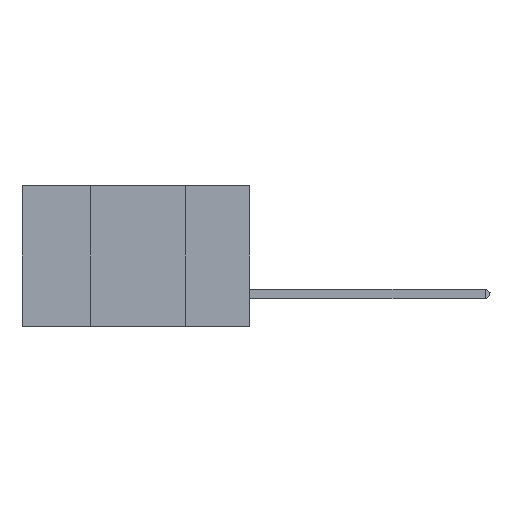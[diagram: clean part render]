
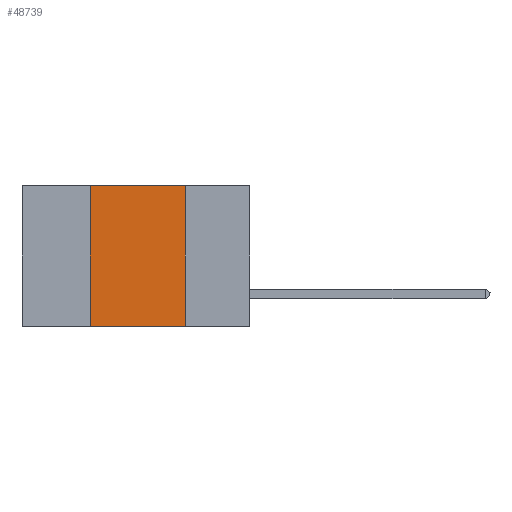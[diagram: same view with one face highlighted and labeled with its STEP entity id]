
A CAD part, left-side view. The second image highlights one B-rep face of the part: STEP entity #48739.
In plain terms, the highlighted planar face has unit normal (-1, 0, 0).
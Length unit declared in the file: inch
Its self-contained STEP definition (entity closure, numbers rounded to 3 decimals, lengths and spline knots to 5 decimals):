
#16 = LINE ( 'NONE', #6205, #40571 ) ;
#201 = CARTESIAN_POINT ( 'NONE',  ( 0., 0.6, 0. ) ) ;
#2793 = DIRECTION ( 'NONE',  ( 0., -1., 0. ) ) ;
#3436 = CARTESIAN_POINT ( 'NONE',  ( 0., 0.6, -0.37 ) ) ;
#4112 = PLANE ( 'NONE',  #21368 ) ;
#5822 = VERTEX_POINT ( 'NONE', #38594 ) ;
#6057 = ORIENTED_EDGE ( 'NONE', *, *, #24401, .F. ) ;
#6205 = CARTESIAN_POINT ( 'NONE',  ( 0., 0.6, 0. ) ) ;
#8920 = CARTESIAN_POINT ( 'NONE',  ( 0., 0.17, -0.37 ) ) ;
#11602 = CARTESIAN_POINT ( 'NONE',  ( 0., 0.17, 0. ) ) ;
#15318 = LINE ( 'NONE', #11602, #41174 ) ;
#19025 = DIRECTION ( 'NONE',  ( 0., 0., -1. ) ) ;
#19701 = VERTEX_POINT ( 'NONE', #44181 ) ;
#20139 = VERTEX_POINT ( 'NONE', #31394 ) ;
#20397 = DIRECTION ( 'NONE',  ( 1., 0., 0. ) ) ;
#21368 = AXIS2_PLACEMENT_3D ( 'NONE', #201, #20397, #40037 ) ;
#21485 = LINE ( 'NONE', #29884, #40551 ) ;
#23314 = LINE ( 'NONE', #3436, #45417 ) ;
#24401 = EDGE_CURVE ( 'NONE', #20139, #5822, #21485, .T. ) ;
#25760 = DIRECTION ( 'NONE',  ( 0., 0., 1. ) ) ;
#25845 = FACE_OUTER_BOUND ( 'NONE', #41307, .T. ) ;
#26761 = EDGE_CURVE ( 'NONE', #20139, #47123, #23314, .T. ) ;
#27064 = ORIENTED_EDGE ( 'NONE', *, *, #38876, .F. ) ;
#29884 = CARTESIAN_POINT ( 'NONE',  ( 0., 0.42, 0. ) ) ;
#31394 = CARTESIAN_POINT ( 'NONE',  ( 0., 0.42, -0.37 ) ) ;
#33507 = ORIENTED_EDGE ( 'NONE', *, *, #26761, .T. ) ;
#38249 = ORIENTED_EDGE ( 'NONE', *, *, #39695, .F. ) ;
#38315 = DIRECTION ( 'NONE',  ( 0., -1., 0. ) ) ;
#38594 = CARTESIAN_POINT ( 'NONE',  ( 0., 0.42, 0. ) ) ;
#38876 = EDGE_CURVE ( 'NONE', #5822, #19701, #16, .T. ) ;
#39695 = EDGE_CURVE ( 'NONE', #19701, #47123, #15318, .T. ) ;
#40037 = DIRECTION ( 'NONE',  ( 0., 0., -1. ) ) ;
#40551 = VECTOR ( 'NONE', #25760, 39.37008 ) ;
#40571 = VECTOR ( 'NONE', #2793, 39.37008 ) ;
#41174 = VECTOR ( 'NONE', #19025, 39.37008 ) ;
#41307 = EDGE_LOOP ( 'NONE', ( #38249, #27064, #6057, #33507 ) ) ;
#44181 = CARTESIAN_POINT ( 'NONE',  ( 0., 0.17, 0. ) ) ;
#45417 = VECTOR ( 'NONE', #38315, 39.37008 ) ;
#47123 = VERTEX_POINT ( 'NONE', #8920 ) ;
#48739 = ADVANCED_FACE ( 'NONE', ( #25845 ), #4112, .F. ) ;
